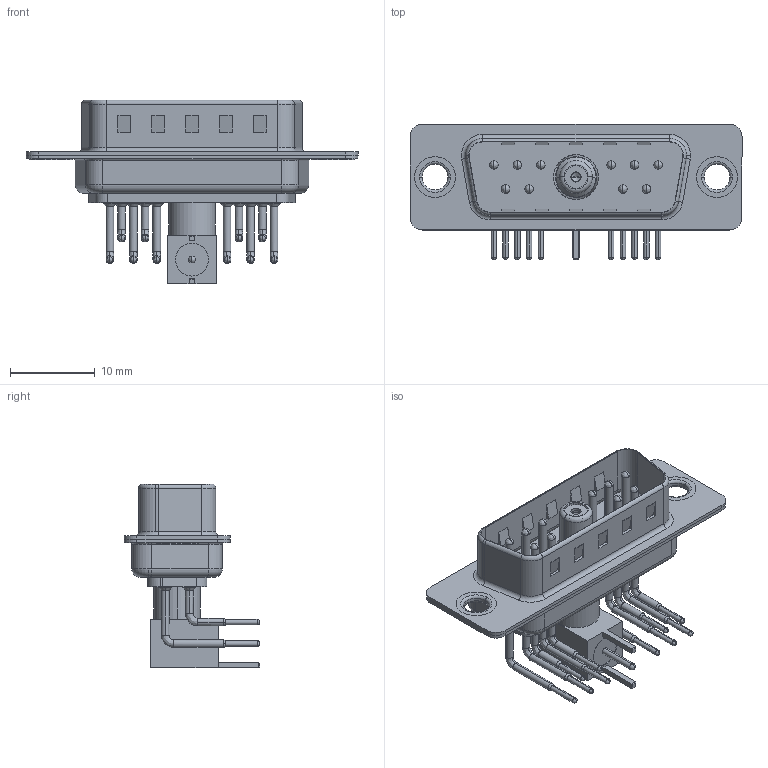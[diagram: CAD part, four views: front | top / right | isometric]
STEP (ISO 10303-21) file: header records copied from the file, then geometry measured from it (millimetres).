
FILE_DESCRIPTION (( 'STEP AP203' ), '1' );
FILE_NAME ('629-11W1240-7N1.STEP', '2022-05-06T21:44:02', ( '' ), ( '' ), 'SwSTEP 2.0', 'SolidWorks 2020', '' );
FILE_SCHEMA (( 'CONFIG_CONTROL_DESIGN' ));
Length unit declared in the file: millimetre
Products named in the file (15): 629Combo Thru Hole Rivet; Insulator Socket; 629Combo Shell Front_15 Contacts; 629Combo Shell Rear_15 Contacts; Socket_RA; Insulator RA Pin; Co-Ax Jack_RA PC Tail; 629Combo Contact Row 2; 629Combo Contact Row 1; 629-11W1240-7N1; Co-Ax Jack Assy_RA; Locking Collar; RA Back Shell; Insulator Socket 2; 629Combo Housing_11W1
Assembly tree (23 placements, depth 3):
  629-11W1240-7N1
    629Combo Housing_11W1
    629Combo Shell Rear_15 Contacts
    629Combo Shell Front_15 Contacts
    629Combo Thru Hole Rivet  x2
    Co-Ax Jack Assy_RA
      Co-Ax Jack_RA PC Tail
      Insulator Socket
      Insulator Socket 2
      Locking Collar
      Socket_RA
      RA Back Shell
      Insulator RA Pin
    629Combo Contact Row 1  x6
    629Combo Contact Row 2  x4
Bounding box: 39.2 x 16 x 21.71 mm (x, y, z)
Volume: 2134.2 mm3; surface area: 5932.7 mm2
Topology: 22 solids, 25 shells, 1579 faces, 4253 edges, 2741 vertices
Faces by surface type: plane 845, cylinder 548, torus 64, bspline 61, cone 59, sphere 2
Entity records: 24485 total; most frequent: CARTESIAN_POINT 4241, DIRECTION 4052, ORIENTED_EDGE 3694, EDGE_CURVE 1847, AXIS2_PLACEMENT_3D 1481, VERTEX_POINT 1185, LINE 1090, VECTOR 1090
